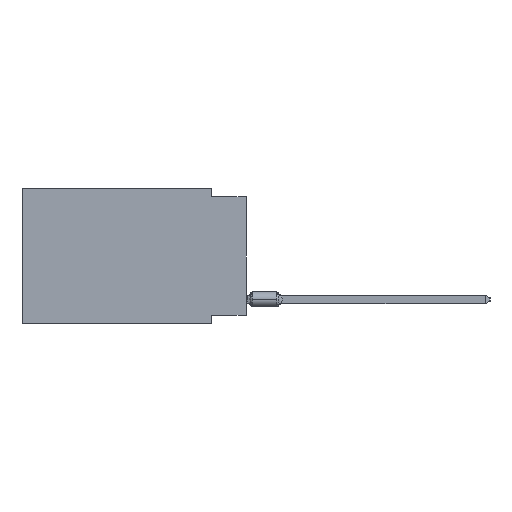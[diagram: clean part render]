
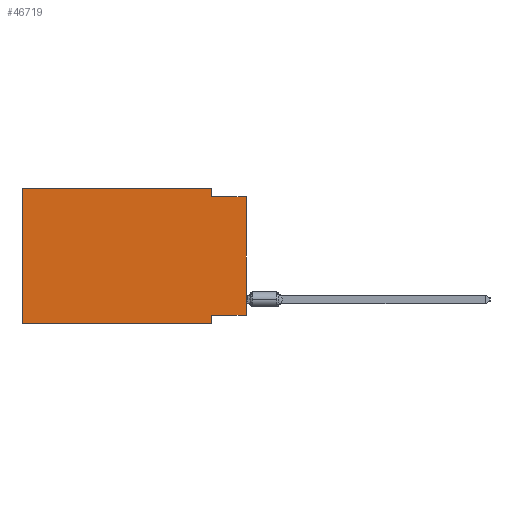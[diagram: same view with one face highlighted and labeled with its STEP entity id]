
A CAD part, left-side view. The second image highlights one B-rep face of the part: STEP entity #46719.
In plain terms, the highlighted planar face has unit normal (-1, 0, 0).
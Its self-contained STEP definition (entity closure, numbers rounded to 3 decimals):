
#179 = ORIENTED_EDGE ( 'NONE', *, *, #61760, .F. ) ;
#245 = CARTESIAN_POINT ( 'NONE',  ( 0., 2.54, -9.271 ) ) ;
#1828 = CARTESIAN_POINT ( 'NONE',  ( 0., 2.54, -0.635 ) ) ;
#2715 = LINE ( 'NONE', #8301, #12263 ) ;
#3768 = VECTOR ( 'NONE', #14468, 1000. ) ;
#3948 = LINE ( 'NONE', #19960, #27678 ) ;
#3998 = DIRECTION ( 'NONE',  ( 0., 0., -1. ) ) ;
#4190 = DIRECTION ( 'NONE',  ( 0., 0., 1. ) ) ;
#8301 = CARTESIAN_POINT ( 'NONE',  ( 0., 16.383, 0. ) ) ;
#9109 = VECTOR ( 'NONE', #12214, 1000. ) ;
#9544 = ORIENTED_EDGE ( 'NONE', *, *, #27073, .F. ) ;
#9600 = DIRECTION ( 'NONE',  ( 0., -1., 0. ) ) ;
#9940 = LINE ( 'NONE', #30161, #28442 ) ;
#10225 = CARTESIAN_POINT ( 'NONE',  ( 0., 0., -9.271 ) ) ;
#10503 = VERTEX_POINT ( 'NONE', #63281 ) ;
#12132 = ORIENTED_EDGE ( 'NONE', *, *, #19218, .T. ) ;
#12214 = DIRECTION ( 'NONE',  ( 0., -1., 0. ) ) ;
#12263 = VECTOR ( 'NONE', #51174, 1000. ) ;
#14468 = DIRECTION ( 'NONE',  ( 0., 0., -1. ) ) ;
#16993 = CARTESIAN_POINT ( 'NONE',  ( 0., 2.54, -9.906 ) ) ;
#18178 = CARTESIAN_POINT ( 'NONE',  ( 0., 16.383, -9.906 ) ) ;
#18918 = EDGE_CURVE ( 'NONE', #44307, #38059, #9940, .T. ) ;
#19005 = LINE ( 'NONE', #25278, #3768 ) ;
#19218 = EDGE_CURVE ( 'NONE', #59977, #10503, #35248, .T. ) ;
#19330 = CARTESIAN_POINT ( 'NONE',  ( 0., 2.54, -9.906 ) ) ;
#19960 = CARTESIAN_POINT ( 'NONE',  ( 0., 16.383, 0. ) ) ;
#20213 = DIRECTION ( 'NONE',  ( 0., 1., 0. ) ) ;
#21998 = EDGE_CURVE ( 'NONE', #59977, #48914, #40831, .T. ) ;
#25278 = CARTESIAN_POINT ( 'NONE',  ( 0., 2.54, 0. ) ) ;
#25429 = ORIENTED_EDGE ( 'NONE', *, *, #21998, .F. ) ;
#25724 = PLANE ( 'NONE',  #33276 ) ;
#27073 = EDGE_CURVE ( 'NONE', #64213, #41464, #19005, .T. ) ;
#27678 = VECTOR ( 'NONE', #31115, 1000. ) ;
#28442 = VECTOR ( 'NONE', #9600, 1000. ) ;
#30161 = CARTESIAN_POINT ( 'NONE',  ( 0., 16.383, -9.906 ) ) ;
#31115 = DIRECTION ( 'NONE',  ( 0., 0., 1. ) ) ;
#32736 = EDGE_CURVE ( 'NONE', #66230, #64213, #2715, .T. ) ;
#33276 = AXIS2_PLACEMENT_3D ( 'NONE', #68588, #36198, #47686 ) ;
#35248 = LINE ( 'NONE', #51973, #40768 ) ;
#36198 = DIRECTION ( 'NONE',  ( 1., 0., 0. ) ) ;
#37524 = ORIENTED_EDGE ( 'NONE', *, *, #46314, .F. ) ;
#38059 = VERTEX_POINT ( 'NONE', #16993 ) ;
#38728 = LINE ( 'NONE', #59969, #9109 ) ;
#40768 = VECTOR ( 'NONE', #4190, 1000. ) ;
#40831 = LINE ( 'NONE', #45726, #66805 ) ;
#41464 = VERTEX_POINT ( 'NONE', #1828 ) ;
#42764 = EDGE_LOOP ( 'NONE', ( #12132, #179, #9544, #45355, #37524, #53971, #54088, #25429 ) ) ;
#44307 = VERTEX_POINT ( 'NONE', #18178 ) ;
#45355 = ORIENTED_EDGE ( 'NONE', *, *, #32736, .F. ) ;
#45726 = CARTESIAN_POINT ( 'NONE',  ( 0., 0., -9.271 ) ) ;
#46218 = LINE ( 'NONE', #19330, #57028 ) ;
#46314 = EDGE_CURVE ( 'NONE', #44307, #66230, #3948, .T. ) ;
#46719 = ADVANCED_FACE ( 'NONE', ( #52917 ), #25724, .F. ) ;
#47686 = DIRECTION ( 'NONE',  ( 0., 0., -1. ) ) ;
#48914 = VERTEX_POINT ( 'NONE', #245 ) ;
#51174 = DIRECTION ( 'NONE',  ( 0., -1., 0. ) ) ;
#51973 = CARTESIAN_POINT ( 'NONE',  ( 0., 0., 0. ) ) ;
#52917 = FACE_OUTER_BOUND ( 'NONE', #42764, .T. ) ;
#53971 = ORIENTED_EDGE ( 'NONE', *, *, #18918, .T. ) ;
#54088 = ORIENTED_EDGE ( 'NONE', *, *, #63756, .F. ) ;
#57028 = VECTOR ( 'NONE', #3998, 1000. ) ;
#59969 = CARTESIAN_POINT ( 'NONE',  ( 0., 0., -0.635 ) ) ;
#59977 = VERTEX_POINT ( 'NONE', #10225 ) ;
#61760 = EDGE_CURVE ( 'NONE', #41464, #10503, #38728, .T. ) ;
#62113 = CARTESIAN_POINT ( 'NONE',  ( 0., 2.54, 0. ) ) ;
#63281 = CARTESIAN_POINT ( 'NONE',  ( 0., 0., -0.635 ) ) ;
#63756 = EDGE_CURVE ( 'NONE', #48914, #38059, #46218, .T. ) ;
#64213 = VERTEX_POINT ( 'NONE', #62113 ) ;
#64788 = CARTESIAN_POINT ( 'NONE',  ( 0., 16.383, 0. ) ) ;
#66230 = VERTEX_POINT ( 'NONE', #64788 ) ;
#66805 = VECTOR ( 'NONE', #20213, 1000. ) ;
#68588 = CARTESIAN_POINT ( 'NONE',  ( 0., 16.383, 0. ) ) ;
